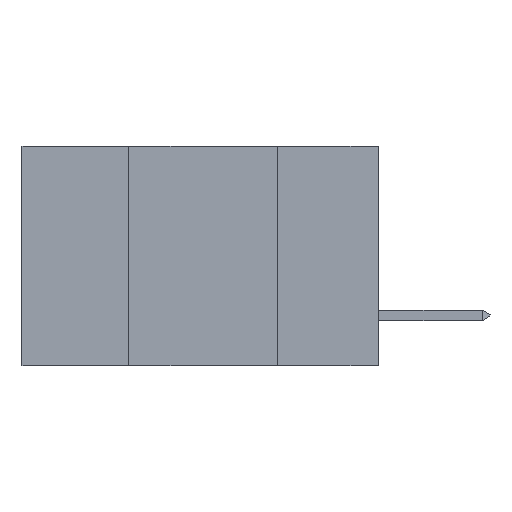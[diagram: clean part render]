
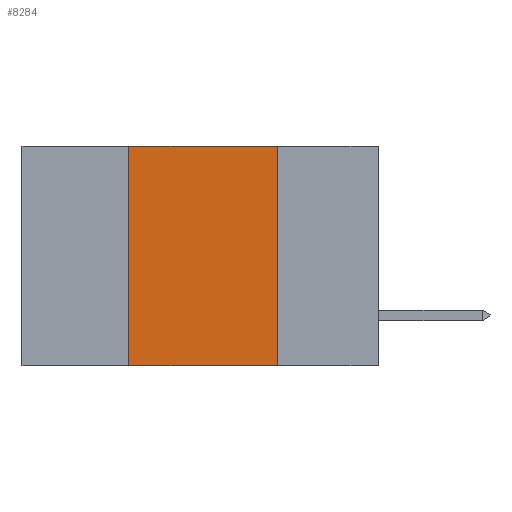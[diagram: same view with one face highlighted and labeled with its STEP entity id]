
A CAD part, left-side view. The second image highlights one B-rep face of the part: STEP entity #8284.
In plain terms, the highlighted planar face has unit normal (-1, 0, 0).
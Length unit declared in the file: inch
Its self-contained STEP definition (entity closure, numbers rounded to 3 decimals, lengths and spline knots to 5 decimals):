
#44 = VECTOR ( 'NONE', #3887, 39.37008 ) ;
#376 = CARTESIAN_POINT ( 'NONE',  ( 0., 0.42, 0. ) ) ;
#823 = DIRECTION ( 'NONE',  ( 0., 0., 1. ) ) ;
#1098 = VERTEX_POINT ( 'NONE', #3327 ) ;
#1688 = CARTESIAN_POINT ( 'NONE',  ( 0., 0.6, -0.37 ) ) ;
#1768 = EDGE_CURVE ( 'NONE', #12019, #9109, #4535, .T. ) ;
#2032 = ORIENTED_EDGE ( 'NONE', *, *, #5942, .F. ) ;
#2474 = AXIS2_PLACEMENT_3D ( 'NONE', #11238, #7415, #9185 ) ;
#2570 = CARTESIAN_POINT ( 'NONE',  ( 0., 0.17, 0. ) ) ;
#2675 = ORIENTED_EDGE ( 'NONE', *, *, #8920, .F. ) ;
#3024 = CARTESIAN_POINT ( 'NONE',  ( 0., 0.6, 0. ) ) ;
#3327 = CARTESIAN_POINT ( 'NONE',  ( 0., 0.17, 0. ) ) ;
#3417 = LINE ( 'NONE', #2570, #3851 ) ;
#3851 = VECTOR ( 'NONE', #8344, 39.37008 ) ;
#3887 = DIRECTION ( 'NONE',  ( 0., -1., 0. ) ) ;
#4531 = PLANE ( 'NONE',  #2474 ) ;
#4535 = LINE ( 'NONE', #12164, #10722 ) ;
#4540 = EDGE_LOOP ( 'NONE', ( #2032, #2675, #8874, #6331 ) ) ;
#4607 = VECTOR ( 'NONE', #11527, 39.37008 ) ;
#5942 = EDGE_CURVE ( 'NONE', #1098, #9726, #3417, .T. ) ;
#6005 = CARTESIAN_POINT ( 'NONE',  ( 0., 0.17, -0.37 ) ) ;
#6331 = ORIENTED_EDGE ( 'NONE', *, *, #10872, .T. ) ;
#7285 = LINE ( 'NONE', #1688, #4607 ) ;
#7415 = DIRECTION ( 'NONE',  ( 1., 0., 0. ) ) ;
#7840 = FACE_OUTER_BOUND ( 'NONE', #4540, .T. ) ;
#8284 = ADVANCED_FACE ( 'NONE', ( #7840 ), #4531, .F. ) ;
#8297 = CARTESIAN_POINT ( 'NONE',  ( 0., 0.42, -0.37 ) ) ;
#8344 = DIRECTION ( 'NONE',  ( 0., 0., -1. ) ) ;
#8874 = ORIENTED_EDGE ( 'NONE', *, *, #1768, .F. ) ;
#8920 = EDGE_CURVE ( 'NONE', #9109, #1098, #9744, .T. ) ;
#9109 = VERTEX_POINT ( 'NONE', #376 ) ;
#9185 = DIRECTION ( 'NONE',  ( 0., 0., -1. ) ) ;
#9726 = VERTEX_POINT ( 'NONE', #6005 ) ;
#9744 = LINE ( 'NONE', #3024, #44 ) ;
#10722 = VECTOR ( 'NONE', #823, 39.37008 ) ;
#10872 = EDGE_CURVE ( 'NONE', #12019, #9726, #7285, .T. ) ;
#11238 = CARTESIAN_POINT ( 'NONE',  ( 0., 0.6, 0. ) ) ;
#11527 = DIRECTION ( 'NONE',  ( 0., -1., 0. ) ) ;
#12019 = VERTEX_POINT ( 'NONE', #8297 ) ;
#12164 = CARTESIAN_POINT ( 'NONE',  ( 0., 0.42, 0. ) ) ;
